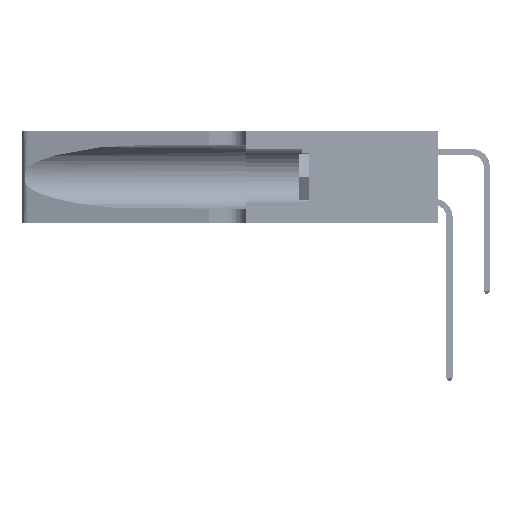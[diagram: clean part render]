
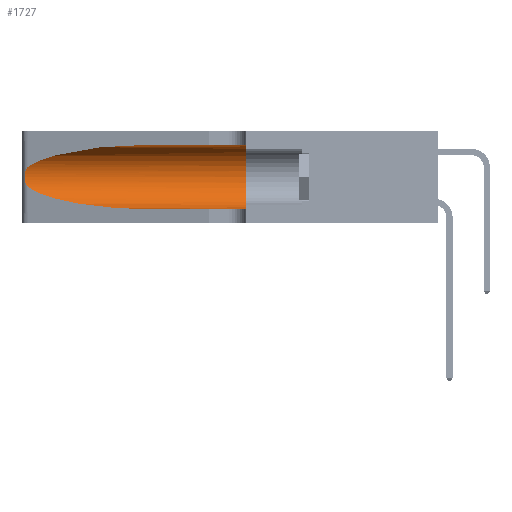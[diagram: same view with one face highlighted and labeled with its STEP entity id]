
A CAD part, left-side view. The second image highlights one B-rep face of the part: STEP entity #1727.
In plain terms, the highlighted cylindrical face has radius 3.308 mm (diameter 6.617 mm), a partial arc.
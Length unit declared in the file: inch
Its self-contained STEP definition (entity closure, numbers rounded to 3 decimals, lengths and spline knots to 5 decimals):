
#1727 = ADVANCED_FACE ( 'NONE', ( #38143 ), #36976, .F. ) ;
#2087 = CARTESIAN_POINT ( 'NONE',  ( 0.25487, 1.22718, 0.22369 ) ) ;
#2118 = VECTOR ( 'NONE', #28599, 39.37008 ) ;
#2491 = ORIENTED_EDGE ( 'NONE', *, *, #21548, .F. ) ;
#3212 = EDGE_CURVE ( 'NONE', #24578, #31329, #25750, .T. ) ;
#3921 = EDGE_CURVE ( 'NONE', #31329, #4022, #4534, .T. ) ;
#4022 = VERTEX_POINT ( 'NONE', #32878 ) ;
#4218 = CARTESIAN_POINT ( 'NONE',  ( 0.25787, 1.23484, 0.2124 ) ) ;
#4534 = LINE ( 'NONE', #9861, #2118 ) ;
#4880 = EDGE_CURVE ( 'NONE', #11858, #24578, #17025, .T. ) ;
#5010 = DIRECTION ( 'NONE',  ( 0., -1., 0. ) ) ;
#5088 = VERTEX_POINT ( 'NONE', #39162 ) ;
#7180 = CARTESIAN_POINT ( 'NONE',  ( 0.1305, 0.35, 0.185 ) ) ;
#8016 = CARTESIAN_POINT ( 'NONE',  ( 0.26018, 1.23835, 0.19895 ) ) ;
#9757 = CARTESIAN_POINT ( 'NONE',  ( 0.1305, 0.72297, 0.05475 ) ) ;
#9861 = CARTESIAN_POINT ( 'NONE',  ( 0.1305, 1.61858, 0.05475 ) ) ;
#10037 = CIRCLE ( 'NONE', #21006, 0.13025 ) ;
#10591 = VECTOR ( 'NONE', #48507, 39.37008 ) ;
#10929 = DIRECTION ( 'NONE',  ( 0., 0., 1. ) ) ;
#11778 = CARTESIAN_POINT ( 'NONE',  ( 0.26075, 1.23896, 0.178 ) ) ;
#11858 = VERTEX_POINT ( 'NONE', #17754 ) ;
#12593 = VERTEX_POINT ( 'NONE', #22457 ) ;
#15565 = CARTESIAN_POINT ( 'NONE',  ( 0.25856, 1.23593, 0.16098 ) ) ;
#17025 = B_SPLINE_CURVE_WITH_KNOTS ( 'NONE', 3,
 ( #45347, #19177, #26737, #4218, #30506, #8016, #34297, #11778, #38019, #15565, #41766, #19335, #45505, #23085 ),
 .UNSPECIFIED., .F., .F.,
 ( 4, 2, 2, 2, 2, 2, 4 ),
 ( 0., 0.00027, 0.00053, 0.00107, 0.0016, 0.00187, 0.00214 ),
 .UNSPECIFIED. ) ;
#17108 = EDGE_LOOP ( 'NONE', ( #18021, #40930, #17840, #18601, #29768, #2491 ) ) ;
#17754 = CARTESIAN_POINT ( 'NONE',  ( 0.25487, 1.22718, 0.22369 ) ) ;
#17840 = ORIENTED_EDGE ( 'NONE', *, *, #3212, .T. ) ;
#18021 = ORIENTED_EDGE ( 'NONE', *, *, #35397, .T. ) ;
#18601 = ORIENTED_EDGE ( 'NONE', *, *, #3921, .T. ) ;
#19177 = CARTESIAN_POINT ( 'NONE',  ( 0.25555, 1.22994, 0.2215 ) ) ;
#19335 = CARTESIAN_POINT ( 'NONE',  ( 0.25639, 1.23186, 0.15144 ) ) ;
#19910 = DIRECTION ( 'NONE',  ( 0., 0., -1. ) ) ;
#20836 = CARTESIAN_POINT ( 'NONE',  ( 0.1305, 0.72297, 0.31525 ) ) ;
#21006 = AXIS2_PLACEMENT_3D ( 'NONE', #7180, #33451, #10929 ) ;
#21160 = CARTESIAN_POINT ( 'NONE',  ( 0.25487, 1.22718, 0.14631 ) ) ;
#21548 = EDGE_CURVE ( 'NONE', #5088, #12593, #48098, .T. ) ;
#22457 = CARTESIAN_POINT ( 'NONE',  ( 0.1305, 0.35, 0.31525 ) ) ;
#23085 = CARTESIAN_POINT ( 'NONE',  ( 0.25487, 1.22718, 0.14631 ) ) ;
#24578 = VERTEX_POINT ( 'NONE', #21160 ) ;
#24616 = CARTESIAN_POINT ( 'NONE',  ( 0.2373, 1.15595, 0.28018 ) ) ;
#25750 =( BOUNDED_CURVE ( )  B_SPLINE_CURVE ( 3, ( #32277, #28331, #28492, #9757 ),
 .UNSPECIFIED., .F., .F. ) 
 B_SPLINE_CURVE_WITH_KNOTS ( ( 4, 4 ),
 ( 3.44316, 4.71239 ),
 .UNSPECIFIED. ) 
 CURVE ( )  GEOMETRIC_REPRESENTATION_ITEM ( )  RATIONAL_B_SPLINE_CURVE ( ( 1., 0.87, 0.87, 1. ) ) 
 REPRESENTATION_ITEM ( '' )  );
#26737 = CARTESIAN_POINT ( 'NONE',  ( 0.25639, 1.23184, 0.21858 ) ) ;
#28331 = CARTESIAN_POINT ( 'NONE',  ( 0.2373, 1.15595, 0.08982 ) ) ;
#28492 = CARTESIAN_POINT ( 'NONE',  ( 0.18966, 0.96281, 0.05475 ) ) ;
#28599 = DIRECTION ( 'NONE',  ( 0., -1., 0. ) ) ;
#29768 = ORIENTED_EDGE ( 'NONE', *, *, #30911, .F. ) ;
#30506 = CARTESIAN_POINT ( 'NONE',  ( 0.25854, 1.2359, 0.20912 ) ) ;
#30911 = EDGE_CURVE ( 'NONE', #12593, #4022, #10037, .T. ) ;
#31329 = VERTEX_POINT ( 'NONE', #43718 ) ;
#32277 = CARTESIAN_POINT ( 'NONE',  ( 0.25487, 1.22718, 0.14631 ) ) ;
#32878 = CARTESIAN_POINT ( 'NONE',  ( 0.1305, 0.35, 0.05475 ) ) ;
#33451 = DIRECTION ( 'NONE',  ( 0., 1., 0. ) ) ;
#34297 = CARTESIAN_POINT ( 'NONE',  ( 0.26075, 1.23896, 0.19203 ) ) ;
#35397 = EDGE_CURVE ( 'NONE', #5088, #11858, #35981, .T. ) ;
#35981 =( BOUNDED_CURVE ( )  B_SPLINE_CURVE ( 3, ( #20836, #47024, #24616, #2087 ),
 .UNSPECIFIED., .F., .T. ) 
 B_SPLINE_CURVE_WITH_KNOTS ( ( 4, 4 ),
 ( 1.5708, 2.84003 ),
 .UNSPECIFIED. ) 
 CURVE ( )  GEOMETRIC_REPRESENTATION_ITEM ( )  RATIONAL_B_SPLINE_CURVE ( ( 1., 0.87, 0.87, 1. ) ) 
 REPRESENTATION_ITEM ( '' )  );
#36976 = CYLINDRICAL_SURFACE ( 'NONE', #43234, 0.13025 ) ;
#38019 = CARTESIAN_POINT ( 'NONE',  ( 0.26017, 1.23833, 0.17102 ) ) ;
#38143 = FACE_OUTER_BOUND ( 'NONE', #17108, .T. ) ;
#39162 = CARTESIAN_POINT ( 'NONE',  ( 0.1305, 0.72297, 0.31525 ) ) ;
#40930 = ORIENTED_EDGE ( 'NONE', *, *, #4880, .T. ) ;
#41766 = CARTESIAN_POINT ( 'NONE',  ( 0.25789, 1.23486, 0.15765 ) ) ;
#43234 = AXIS2_PLACEMENT_3D ( 'NONE', #46092, #5010, #19910 ) ;
#43718 = CARTESIAN_POINT ( 'NONE',  ( 0.1305, 0.72297, 0.05475 ) ) ;
#44771 = CARTESIAN_POINT ( 'NONE',  ( 0.1305, 1.61858, 0.31525 ) ) ;
#45347 = CARTESIAN_POINT ( 'NONE',  ( 0.25487, 1.22718, 0.22369 ) ) ;
#45505 = CARTESIAN_POINT ( 'NONE',  ( 0.25555, 1.22993, 0.14849 ) ) ;
#46092 = CARTESIAN_POINT ( 'NONE',  ( 0.1305, 1.61858, 0.185 ) ) ;
#47024 = CARTESIAN_POINT ( 'NONE',  ( 0.18966, 0.96281, 0.31525 ) ) ;
#48098 = LINE ( 'NONE', #44771, #10591 ) ;
#48507 = DIRECTION ( 'NONE',  ( 0., -1., 0. ) ) ;
